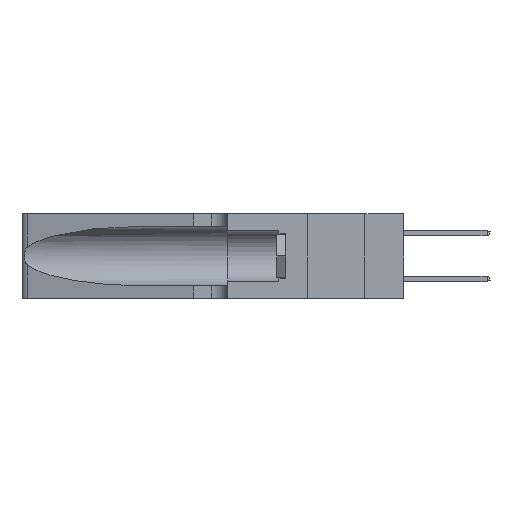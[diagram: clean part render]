
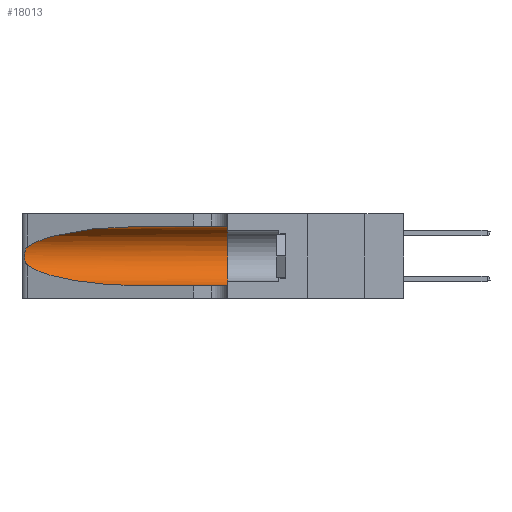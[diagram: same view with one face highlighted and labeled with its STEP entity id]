
A CAD part, left-side view. The second image highlights one B-rep face of the part: STEP entity #18013.
In plain terms, the highlighted cylindrical face has radius 3.308 mm (diameter 6.617 mm), a partial arc.
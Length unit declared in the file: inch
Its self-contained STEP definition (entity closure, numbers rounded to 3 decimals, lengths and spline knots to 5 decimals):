
#486 = ORIENTED_EDGE ( 'NONE', *, *, #10149, .T. ) ;
#793 = VERTEX_POINT ( 'NONE', #16218 ) ;
#1567 = CARTESIAN_POINT ( 'NONE',  ( 0.1305, 1.61858, 0.05475 ) ) ;
#1995 = CARTESIAN_POINT ( 'NONE',  ( 0.26075, 1.23896, 0.178 ) ) ;
#3619 = VERTEX_POINT ( 'NONE', #6272 ) ;
#3900 = ORIENTED_EDGE ( 'NONE', *, *, #25049, .F. ) ;
#4883 = DIRECTION ( 'NONE',  ( 0., -1., 0. ) ) ;
#5198 = CARTESIAN_POINT ( 'NONE',  ( 0.2373, 1.15595, 0.08982 ) ) ;
#5283 = CARTESIAN_POINT ( 'NONE',  ( 0.25856, 1.23593, 0.16098 ) ) ;
#5903 = CARTESIAN_POINT ( 'NONE',  ( 0.1305, 1.61858, 0.31525 ) ) ;
#5945 = VERTEX_POINT ( 'NONE', #30793 ) ;
#6047 = VECTOR ( 'NONE', #4883, 39.37008 ) ;
#6272 = CARTESIAN_POINT ( 'NONE',  ( 0.1305, 0.72297, 0.31525 ) ) ;
#6848 = DIRECTION ( 'NONE',  ( 0., 1., 0. ) ) ;
#8467 = CARTESIAN_POINT ( 'NONE',  ( 0.18966, 0.96281, 0.05475 ) ) ;
#8550 = CARTESIAN_POINT ( 'NONE',  ( 0.25639, 1.23186, 0.15144 ) ) ;
#8566 = EDGE_CURVE ( 'NONE', #3619, #12622, #13476, .T. ) ;
#8989 = CARTESIAN_POINT ( 'NONE',  ( 0.1305, 1.61858, 0.185 ) ) ;
#9180 = DIRECTION ( 'NONE',  ( 0., -1., 0. ) ) ;
#10100 = CARTESIAN_POINT ( 'NONE',  ( 0.2373, 1.15595, 0.28018 ) ) ;
#10149 = EDGE_CURVE ( 'NONE', #30786, #793, #40294, .T. ) ;
#10353 =( BOUNDED_CURVE ( )  B_SPLINE_CURVE ( 3, ( #24476, #5198, #8467, #30958 ),
 .UNSPECIFIED., .F., .T. ) 
 B_SPLINE_CURVE_WITH_KNOTS ( ( 4, 4 ),
 ( 3.44316, 4.71239 ),
 .UNSPECIFIED. ) 
 CURVE ( )  GEOMETRIC_REPRESENTATION_ITEM ( )  RATIONAL_B_SPLINE_CURVE ( ( 1., 0.87, 0.87, 1. ) ) 
 REPRESENTATION_ITEM ( '' )  );
#10664 = ORIENTED_EDGE ( 'NONE', *, *, #22149, .T. ) ;
#11381 = FACE_OUTER_BOUND ( 'NONE', #18110, .T. ) ;
#11804 = CARTESIAN_POINT ( 'NONE',  ( 0.25487, 1.22718, 0.14631 ) ) ;
#12622 = VERTEX_POINT ( 'NONE', #17072 ) ;
#13476 =( BOUNDED_CURVE ( )  B_SPLINE_CURVE ( 3, ( #38917, #32445, #10100, #32571 ),
 .UNSPECIFIED., .F., .T. ) 
 B_SPLINE_CURVE_WITH_KNOTS ( ( 4, 4 ),
 ( 1.5708, 2.84003 ),
 .UNSPECIFIED. ) 
 CURVE ( )  GEOMETRIC_REPRESENTATION_ITEM ( )  RATIONAL_B_SPLINE_CURVE ( ( 1., 0.87, 0.87, 1. ) ) 
 REPRESENTATION_ITEM ( '' )  );
#13902 = ORIENTED_EDGE ( 'NONE', *, *, #23853, .F. ) ;
#14800 = VERTEX_POINT ( 'NONE', #20212 ) ;
#14918 = CARTESIAN_POINT ( 'NONE',  ( 0.25639, 1.23184, 0.21858 ) ) ;
#16218 = CARTESIAN_POINT ( 'NONE',  ( 0.1305, 0.35, 0.05475 ) ) ;
#17072 = CARTESIAN_POINT ( 'NONE',  ( 0.25487, 1.22718, 0.22369 ) ) ;
#18013 = ADVANCED_FACE ( 'NONE', ( #11381 ), #34993, .F. ) ;
#18110 = EDGE_LOOP ( 'NONE', ( #35046, #41703, #10664, #486, #13902, #3900 ) ) ;
#18137 = CARTESIAN_POINT ( 'NONE',  ( 0.25854, 1.2359, 0.20912 ) ) ;
#19521 = VECTOR ( 'NONE', #9180, 39.37008 ) ;
#20212 = CARTESIAN_POINT ( 'NONE',  ( 0.25487, 1.22718, 0.14631 ) ) ;
#21333 = CARTESIAN_POINT ( 'NONE',  ( 0.26075, 1.23896, 0.19203 ) ) ;
#22149 = EDGE_CURVE ( 'NONE', #14800, #30786, #10353, .T. ) ;
#23853 = EDGE_CURVE ( 'NONE', #5945, #793, #31694, .T. ) ;
#24476 = CARTESIAN_POINT ( 'NONE',  ( 0.25487, 1.22718, 0.14631 ) ) ;
#24554 = CARTESIAN_POINT ( 'NONE',  ( 0.26017, 1.23833, 0.17102 ) ) ;
#25049 = EDGE_CURVE ( 'NONE', #3619, #5945, #29056, .T. ) ;
#25252 = AXIS2_PLACEMENT_3D ( 'NONE', #26104, #6848, #29343 ) ;
#26104 = CARTESIAN_POINT ( 'NONE',  ( 0.1305, 0.35, 0.185 ) ) ;
#27793 = CARTESIAN_POINT ( 'NONE',  ( 0.25789, 1.23486, 0.15765 ) ) ;
#29056 = LINE ( 'NONE', #5903, #19521 ) ;
#29343 = DIRECTION ( 'NONE',  ( 0., 0., 1. ) ) ;
#29674 = B_SPLINE_CURVE_WITH_KNOTS ( 'NONE', 3,
 ( #30902, #34122, #14918, #37364, #18137, #40596, #21333, #1995, #24554, #5283, #27793, #8550, #31035, #11804 ),
 .UNSPECIFIED., .F., .F.,
 ( 4, 2, 2, 2, 2, 2, 4 ),
 ( 0., 0.00027, 0.00053, 0.00107, 0.0016, 0.00187, 0.00214 ),
 .UNSPECIFIED. ) ;
#30786 = VERTEX_POINT ( 'NONE', #38791 ) ;
#30793 = CARTESIAN_POINT ( 'NONE',  ( 0.1305, 0.35, 0.31525 ) ) ;
#30902 = CARTESIAN_POINT ( 'NONE',  ( 0.25487, 1.22718, 0.22369 ) ) ;
#30958 = CARTESIAN_POINT ( 'NONE',  ( 0.1305, 0.72297, 0.05475 ) ) ;
#31035 = CARTESIAN_POINT ( 'NONE',  ( 0.25555, 1.22993, 0.14849 ) ) ;
#31483 = DIRECTION ( 'NONE',  ( 0., -1., 0. ) ) ;
#31694 = CIRCLE ( 'NONE', #25252, 0.13025 ) ;
#32410 = AXIS2_PLACEMENT_3D ( 'NONE', #8989, #31483, #34697 ) ;
#32445 = CARTESIAN_POINT ( 'NONE',  ( 0.18966, 0.96281, 0.31525 ) ) ;
#32571 = CARTESIAN_POINT ( 'NONE',  ( 0.25487, 1.22718, 0.22369 ) ) ;
#34122 = CARTESIAN_POINT ( 'NONE',  ( 0.25555, 1.22994, 0.2215 ) ) ;
#34697 = DIRECTION ( 'NONE',  ( 0., 0., -1. ) ) ;
#34993 = CYLINDRICAL_SURFACE ( 'NONE', #32410, 0.13025 ) ;
#35046 = ORIENTED_EDGE ( 'NONE', *, *, #8566, .T. ) ;
#35401 = EDGE_CURVE ( 'NONE', #12622, #14800, #29674, .T. ) ;
#37364 = CARTESIAN_POINT ( 'NONE',  ( 0.25787, 1.23484, 0.2124 ) ) ;
#38791 = CARTESIAN_POINT ( 'NONE',  ( 0.1305, 0.72297, 0.05475 ) ) ;
#38917 = CARTESIAN_POINT ( 'NONE',  ( 0.1305, 0.72297, 0.31525 ) ) ;
#40294 = LINE ( 'NONE', #1567, #6047 ) ;
#40596 = CARTESIAN_POINT ( 'NONE',  ( 0.26018, 1.23835, 0.19895 ) ) ;
#41703 = ORIENTED_EDGE ( 'NONE', *, *, #35401, .T. ) ;
